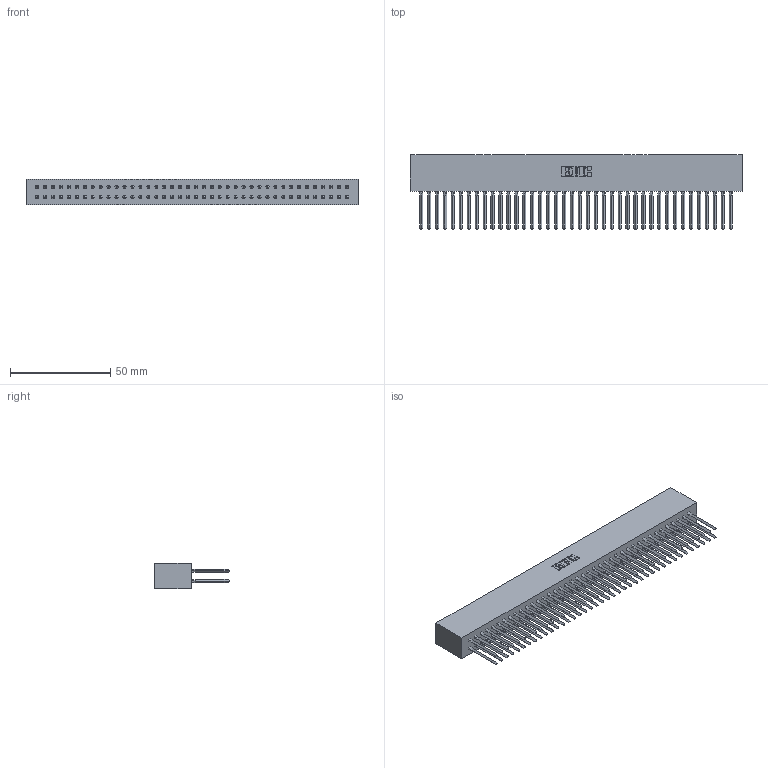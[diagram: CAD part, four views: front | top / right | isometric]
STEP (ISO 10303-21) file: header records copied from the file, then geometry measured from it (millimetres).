
FILE_DESCRIPTION (( 'STEP AP203' ), '1' );
FILE_NAME ('317-080-540-801.STEP', '2020-02-28T09:04:04', ( '' ), ( '' ), 'SwSTEP 2.0', 'SolidWorks 2016', '' );
FILE_SCHEMA (( 'CONFIG_CONTROL_DESIGN' ));
Length unit declared in the file: inch
Products named in the file (3): 317 Part_Lugless; 317-290-001_540; 317-080-540-801
Assembly tree (81 placements, depth 2):
  317-080-540-801
    317 Part_Lugless
    317-290-001_540  x80
Bounding box: 165.71 x 37.34 x 12.7 mm (x, y, z)
Volume: 29537.2 mm3; surface area: 44218.5 mm2
Topology: 81 solids, 81 shells, 7210 faces, 19999 edges, 12878 vertices
Faces by surface type: plane 5890, cylinder 1000, bspline 320
Entity records: 57690 total; most frequent: CARTESIAN_POINT 10479, ORIENTED_EDGE 9978, DIRECTION 8315, EDGE_CURVE 4989, LINE 4741, VECTOR 4741, VERTEX_POINT 3319, AXIS2_PLACEMENT_3D 1787
